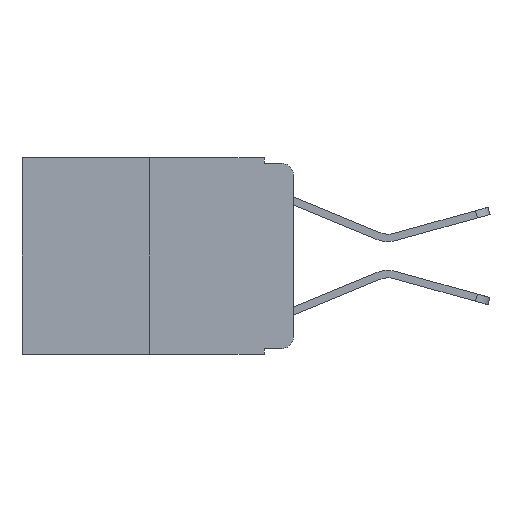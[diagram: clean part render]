
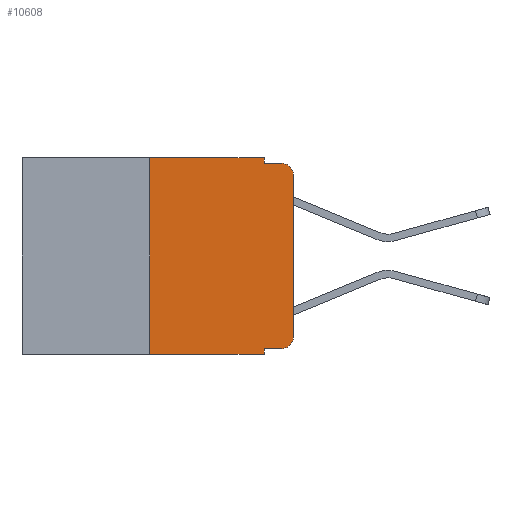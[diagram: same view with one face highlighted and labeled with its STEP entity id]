
A CAD part, left-side view. The second image highlights one B-rep face of the part: STEP entity #10608.
In plain terms, the highlighted planar face has unit normal (-1, 0, 0).
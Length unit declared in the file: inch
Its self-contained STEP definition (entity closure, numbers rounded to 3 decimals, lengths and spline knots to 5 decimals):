
#2 = VECTOR ( 'NONE', #6257, 39.37008 ) ;
#56 = AXIS2_PLACEMENT_3D ( 'NONE', #6732, #10877, #10755 ) ;
#78 = CARTESIAN_POINT ( 'NONE',  ( 0., 0.051, -0.343 ) ) ;
#107 = CARTESIAN_POINT ( 'NONE',  ( 0., 0.051, 0. ) ) ;
#297 = CARTESIAN_POINT ( 'NONE',  ( 0., 0., -0.313 ) ) ;
#381 = VERTEX_POINT ( 'NONE', #6185 ) ;
#465 = DIRECTION ( 'NONE',  ( 0., -1., 0. ) ) ;
#667 = VECTOR ( 'NONE', #2490, 39.37008 ) ;
#759 = VERTEX_POINT ( 'NONE', #78 ) ;
#995 = FACE_OUTER_BOUND ( 'NONE', #7957, .T. ) ;
#1016 = CARTESIAN_POINT ( 'NONE',  ( 0., 0.051, -0.333 ) ) ;
#1312 = EDGE_CURVE ( 'NONE', #12858, #11297, #3026, .T. ) ;
#1389 = LINE ( 'NONE', #8385, #2603 ) ;
#1580 = DIRECTION ( 'NONE',  ( 0., -1., 0. ) ) ;
#1774 = CARTESIAN_POINT ( 'NONE',  ( 0., 0.051, 0. ) ) ;
#1785 = ORIENTED_EDGE ( 'NONE', *, *, #10089, .F. ) ;
#2057 = DIRECTION ( 'NONE',  ( 0., 0., 1. ) ) ;
#2140 = VECTOR ( 'NONE', #465, 39.37008 ) ;
#2223 = CARTESIAN_POINT ( 'NONE',  ( 0., 0.02, -0.01 ) ) ;
#2360 = AXIS2_PLACEMENT_3D ( 'NONE', #3028, #10046, #4002 ) ;
#2481 = VECTOR ( 'NONE', #2057, 39.37008 ) ;
#2490 = DIRECTION ( 'NONE',  ( 0., 0., 1. ) ) ;
#2603 = VECTOR ( 'NONE', #1580, 39.37008 ) ;
#2711 = VECTOR ( 'NONE', #9535, 39.37008 ) ;
#2751 = LINE ( 'NONE', #1774, #11550 ) ;
#2934 = ORIENTED_EDGE ( 'NONE', *, *, #7678, .F. ) ;
#3026 = LINE ( 'NONE', #11026, #2481 ) ;
#3028 = CARTESIAN_POINT ( 'NONE',  ( 0., 0.473, 0. ) ) ;
#3080 = CARTESIAN_POINT ( 'NONE',  ( 0., 0.25, -0.343 ) ) ;
#3110 = EDGE_CURVE ( 'NONE', #7032, #759, #1389, .T. ) ;
#3135 = EDGE_CURVE ( 'NONE', #3506, #12858, #6135, .T. ) ;
#3506 = VERTEX_POINT ( 'NONE', #9362 ) ;
#3667 = CARTESIAN_POINT ( 'NONE',  ( 0., 0.473, 0. ) ) ;
#3739 = ORIENTED_EDGE ( 'NONE', *, *, #3110, .T. ) ;
#3831 = VERTEX_POINT ( 'NONE', #2223 ) ;
#4002 = DIRECTION ( 'NONE',  ( 0., 0., -1. ) ) ;
#4135 = VERTEX_POINT ( 'NONE', #4596 ) ;
#4589 = EDGE_CURVE ( 'NONE', #11297, #3831, #6431, .T. ) ;
#4596 = CARTESIAN_POINT ( 'NONE',  ( 0., 0.051, 0. ) ) ;
#4766 = DIRECTION ( 'NONE',  ( 0., -1., 0. ) ) ;
#4825 = EDGE_CURVE ( 'NONE', #7032, #4854, #11328, .T. ) ;
#4851 = ORIENTED_EDGE ( 'NONE', *, *, #4825, .F. ) ;
#4854 = VERTEX_POINT ( 'NONE', #8558 ) ;
#5190 = ORIENTED_EDGE ( 'NONE', *, *, #10599, .T. ) ;
#5439 = ORIENTED_EDGE ( 'NONE', *, *, #4589, .T. ) ;
#6020 = AXIS2_PLACEMENT_3D ( 'NONE', #10817, #9305, #11013 ) ;
#6135 = CIRCLE ( 'NONE', #56, 0.02 ) ;
#6185 = CARTESIAN_POINT ( 'NONE',  ( 0., 0.051, -0.01 ) ) ;
#6257 = DIRECTION ( 'NONE',  ( 0., 0., -1. ) ) ;
#6431 = CIRCLE ( 'NONE', #6020, 0.02 ) ;
#6493 = CARTESIAN_POINT ( 'NONE',  ( 0., 0.051, -0.01 ) ) ;
#6732 = CARTESIAN_POINT ( 'NONE',  ( 0., 0.02, -0.313 ) ) ;
#7032 = VERTEX_POINT ( 'NONE', #3080 ) ;
#7193 = PLANE ( 'NONE',  #2360 ) ;
#7444 = VERTEX_POINT ( 'NONE', #1016 ) ;
#7446 = CARTESIAN_POINT ( 'NONE',  ( 0., 0.25, 0. ) ) ;
#7481 = LINE ( 'NONE', #6493, #2711 ) ;
#7678 = EDGE_CURVE ( 'NONE', #381, #3831, #7481, .T. ) ;
#7806 = ORIENTED_EDGE ( 'NONE', *, *, #3135, .T. ) ;
#7957 = EDGE_LOOP ( 'NONE', ( #12368, #5439, #2934, #1785, #12351, #4851, #3739, #8637, #5190, #7806 ) ) ;
#8385 = CARTESIAN_POINT ( 'NONE',  ( 0., 0.473, -0.343 ) ) ;
#8558 = CARTESIAN_POINT ( 'NONE',  ( 0., 0.25, 0. ) ) ;
#8617 = VECTOR ( 'NONE', #4766, 39.37008 ) ;
#8637 = ORIENTED_EDGE ( 'NONE', *, *, #11165, .F. ) ;
#9305 = DIRECTION ( 'NONE',  ( -1., 0., 0. ) ) ;
#9362 = CARTESIAN_POINT ( 'NONE',  ( 0., 0.02, -0.333 ) ) ;
#9535 = DIRECTION ( 'NONE',  ( 0., -1., 0. ) ) ;
#9984 = LINE ( 'NONE', #11815, #8617 ) ;
#10046 = DIRECTION ( 'NONE',  ( 1., 0., 0. ) ) ;
#10089 = EDGE_CURVE ( 'NONE', #4135, #381, #2751, .T. ) ;
#10599 = EDGE_CURVE ( 'NONE', #7444, #3506, #9984, .T. ) ;
#10608 = ADVANCED_FACE ( 'NONE', ( #995 ), #7193, .F. ) ;
#10755 = DIRECTION ( 'NONE',  ( 0., 0., -1. ) ) ;
#10795 = EDGE_CURVE ( 'NONE', #4854, #4135, #12654, .T. ) ;
#10817 = CARTESIAN_POINT ( 'NONE',  ( 0., 0.02, -0.03 ) ) ;
#10877 = DIRECTION ( 'NONE',  ( -1., 0., 0. ) ) ;
#11013 = DIRECTION ( 'NONE',  ( 0., 0., -1. ) ) ;
#11026 = CARTESIAN_POINT ( 'NONE',  ( 0., 0., 0. ) ) ;
#11165 = EDGE_CURVE ( 'NONE', #7444, #759, #11264, .T. ) ;
#11264 = LINE ( 'NONE', #107, #2 ) ;
#11297 = VERTEX_POINT ( 'NONE', #11519 ) ;
#11328 = LINE ( 'NONE', #7446, #667 ) ;
#11519 = CARTESIAN_POINT ( 'NONE',  ( 0., 0., -0.03 ) ) ;
#11550 = VECTOR ( 'NONE', #12294, 39.37008 ) ;
#11815 = CARTESIAN_POINT ( 'NONE',  ( 0., 0.051, -0.333 ) ) ;
#12294 = DIRECTION ( 'NONE',  ( 0., 0., -1. ) ) ;
#12351 = ORIENTED_EDGE ( 'NONE', *, *, #10795, .F. ) ;
#12368 = ORIENTED_EDGE ( 'NONE', *, *, #1312, .T. ) ;
#12654 = LINE ( 'NONE', #3667, #2140 ) ;
#12858 = VERTEX_POINT ( 'NONE', #297 ) ;
